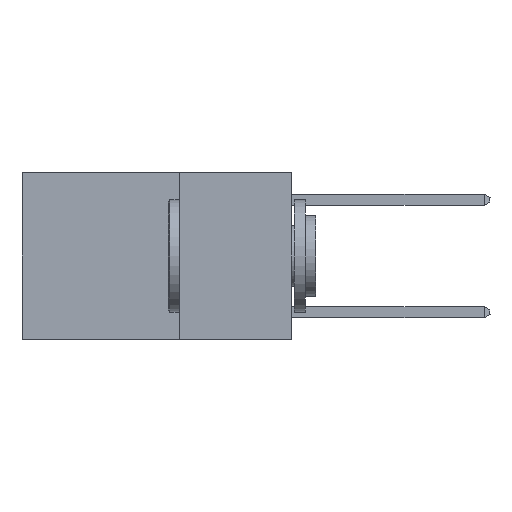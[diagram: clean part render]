
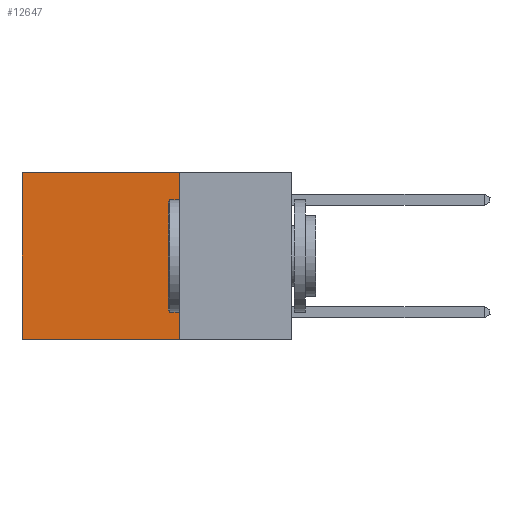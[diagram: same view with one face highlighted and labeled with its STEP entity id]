
A CAD part, left-side view. The second image highlights one B-rep face of the part: STEP entity #12647.
In plain terms, the highlighted planar face has unit normal (-1, 0, 0).
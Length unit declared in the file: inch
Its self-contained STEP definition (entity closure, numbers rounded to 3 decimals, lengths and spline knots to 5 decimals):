
#242 = VECTOR ( 'NONE', #950, 39.37008 ) ;
#594 = CARTESIAN_POINT ( 'NONE',  ( 0.2625, 0.25, 0. ) ) ;
#675 = PLANE ( 'NONE',  #2251 ) ;
#848 = VERTEX_POINT ( 'NONE', #2406 ) ;
#885 = ORIENTED_EDGE ( 'NONE', *, *, #2782, .T. ) ;
#950 = DIRECTION ( 'NONE',  ( 0., 1., 0. ) ) ;
#1178 = DIRECTION ( 'NONE',  ( 0., 0., -1. ) ) ;
#1216 = LINE ( 'NONE', #6048, #12411 ) ;
#1734 = CARTESIAN_POINT ( 'NONE',  ( 0.2625, 0.25, -0.37 ) ) ;
#2251 = AXIS2_PLACEMENT_3D ( 'NONE', #594, #8894, #5340 ) ;
#2406 = CARTESIAN_POINT ( 'NONE',  ( 0.2625, 0.25, -0.37 ) ) ;
#2782 = EDGE_CURVE ( 'NONE', #7094, #6893, #13007, .T. ) ;
#2819 = VECTOR ( 'NONE', #13649, 39.37008 ) ;
#4337 = ORIENTED_EDGE ( 'NONE', *, *, #5146, .T. ) ;
#4418 = LINE ( 'NONE', #1734, #2819 ) ;
#5146 = EDGE_CURVE ( 'NONE', #6893, #15161, #1216, .T. ) ;
#5340 = DIRECTION ( 'NONE',  ( 0., 0., -1. ) ) ;
#6048 = CARTESIAN_POINT ( 'NONE',  ( 0.2625, 0.6, 0. ) ) ;
#6893 = VERTEX_POINT ( 'NONE', #15354 ) ;
#6956 = CARTESIAN_POINT ( 'NONE',  ( 0.2625, 0.25, 0. ) ) ;
#7094 = VERTEX_POINT ( 'NONE', #13069 ) ;
#8420 = EDGE_CURVE ( 'NONE', #7094, #848, #14343, .T. ) ;
#8652 = DIRECTION ( 'NONE',  ( 0., 0., -1. ) ) ;
#8894 = DIRECTION ( 'NONE',  ( 1., 0., 0. ) ) ;
#10900 = CARTESIAN_POINT ( 'NONE',  ( 0.2625, 0.6, -0.37 ) ) ;
#11332 = FACE_OUTER_BOUND ( 'NONE', #14406, .T. ) ;
#11935 = CARTESIAN_POINT ( 'NONE',  ( 0.2625, 0.25, 0. ) ) ;
#12346 = ORIENTED_EDGE ( 'NONE', *, *, #8420, .F. ) ;
#12411 = VECTOR ( 'NONE', #8652, 39.37008 ) ;
#12647 = ADVANCED_FACE ( 'NONE', ( #11332 ), #675, .F. ) ;
#13007 = LINE ( 'NONE', #6956, #242 ) ;
#13069 = CARTESIAN_POINT ( 'NONE',  ( 0.2625, 0.25, 0. ) ) ;
#13603 = VECTOR ( 'NONE', #1178, 39.37008 ) ;
#13649 = DIRECTION ( 'NONE',  ( 0., 1., 0. ) ) ;
#14343 = LINE ( 'NONE', #11935, #13603 ) ;
#14406 = EDGE_LOOP ( 'NONE', ( #4337, #14781, #12346, #885 ) ) ;
#14781 = ORIENTED_EDGE ( 'NONE', *, *, #14848, .F. ) ;
#14848 = EDGE_CURVE ( 'NONE', #848, #15161, #4418, .T. ) ;
#15161 = VERTEX_POINT ( 'NONE', #10900 ) ;
#15354 = CARTESIAN_POINT ( 'NONE',  ( 0.2625, 0.6, 0. ) ) ;
